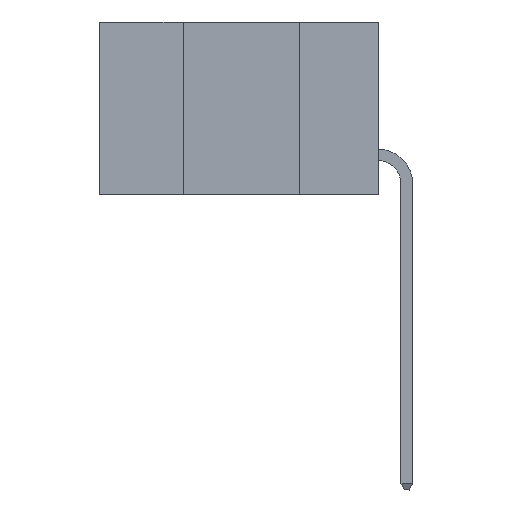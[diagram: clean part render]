
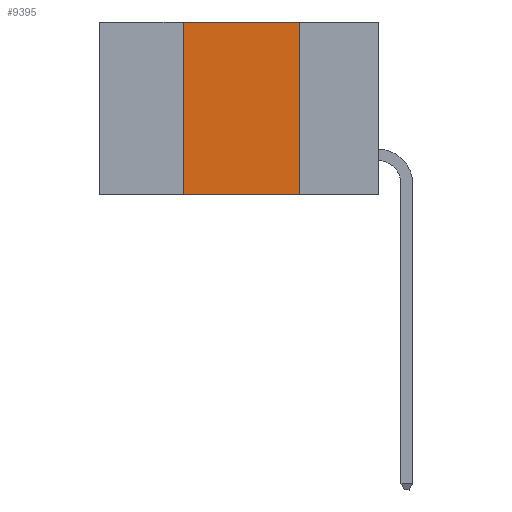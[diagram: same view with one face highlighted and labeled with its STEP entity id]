
A CAD part, left-side view. The second image highlights one B-rep face of the part: STEP entity #9395.
In plain terms, the highlighted planar face has unit normal (-1, 0, 0).
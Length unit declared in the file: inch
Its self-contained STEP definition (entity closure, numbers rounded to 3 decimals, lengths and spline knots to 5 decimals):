
#1109 = DIRECTION ( 'NONE',  ( 0., 0., -1. ) ) ;
#1805 = LINE ( 'NONE', #5755, #12570 ) ;
#2688 = PLANE ( 'NONE',  #4164 ) ;
#4164 = AXIS2_PLACEMENT_3D ( 'NONE', #11761, #13069, #1109 ) ;
#4472 = VERTEX_POINT ( 'NONE', #8813 ) ;
#4918 = LINE ( 'NONE', #8845, #13987 ) ;
#5114 = CARTESIAN_POINT ( 'NONE',  ( 0., 0.6, 0. ) ) ;
#5483 = CARTESIAN_POINT ( 'NONE',  ( 0., 0.17, -0.37 ) ) ;
#5755 = CARTESIAN_POINT ( 'NONE',  ( 0., 0.17, -0.37 ) ) ;
#5920 = EDGE_CURVE ( 'NONE', #9421, #14985, #1805, .T. ) ;
#6760 = LINE ( 'NONE', #5114, #9790 ) ;
#7100 = CARTESIAN_POINT ( 'NONE',  ( 0., 0.42, 0. ) ) ;
#7213 = ORIENTED_EDGE ( 'NONE', *, *, #12065, .T. ) ;
#7754 = FACE_OUTER_BOUND ( 'NONE', #15167, .T. ) ;
#7937 = ORIENTED_EDGE ( 'NONE', *, *, #16586, .F. ) ;
#8291 = DIRECTION ( 'NONE',  ( 0., 0., 1. ) ) ;
#8539 = DIRECTION ( 'NONE',  ( 0., 0., -1. ) ) ;
#8813 = CARTESIAN_POINT ( 'NONE',  ( 0., 0.42, -0.37 ) ) ;
#8845 = CARTESIAN_POINT ( 'NONE',  ( 0., 0.6, -0.37 ) ) ;
#9395 = ADVANCED_FACE ( 'NONE', ( #7754 ), #2688, .F. ) ;
#9421 = VERTEX_POINT ( 'NONE', #17160 ) ;
#9457 = DIRECTION ( 'NONE',  ( 0., -1., 0. ) ) ;
#9790 = VECTOR ( 'NONE', #9457, 39.37008 ) ;
#11761 = CARTESIAN_POINT ( 'NONE',  ( 0., 0.6, 0. ) ) ;
#11807 = EDGE_CURVE ( 'NONE', #11955, #9421, #6760, .T. ) ;
#11955 = VERTEX_POINT ( 'NONE', #7100 ) ;
#12065 = EDGE_CURVE ( 'NONE', #4472, #14985, #4918, .T. ) ;
#12570 = VECTOR ( 'NONE', #8539, 39.37008 ) ;
#13069 = DIRECTION ( 'NONE',  ( 1., 0., 0. ) ) ;
#13207 = VECTOR ( 'NONE', #8291, 39.37008 ) ;
#13603 = CARTESIAN_POINT ( 'NONE',  ( 0., 0.42, -0.37 ) ) ;
#13912 = DIRECTION ( 'NONE',  ( 0., -1., 0. ) ) ;
#13987 = VECTOR ( 'NONE', #13912, 39.37008 ) ;
#14126 = ORIENTED_EDGE ( 'NONE', *, *, #5920, .F. ) ;
#14764 = ORIENTED_EDGE ( 'NONE', *, *, #11807, .F. ) ;
#14985 = VERTEX_POINT ( 'NONE', #5483 ) ;
#15167 = EDGE_LOOP ( 'NONE', ( #14126, #14764, #7937, #7213 ) ) ;
#16473 = LINE ( 'NONE', #13603, #13207 ) ;
#16586 = EDGE_CURVE ( 'NONE', #4472, #11955, #16473, .T. ) ;
#17160 = CARTESIAN_POINT ( 'NONE',  ( 0., 0.17, 0. ) ) ;
